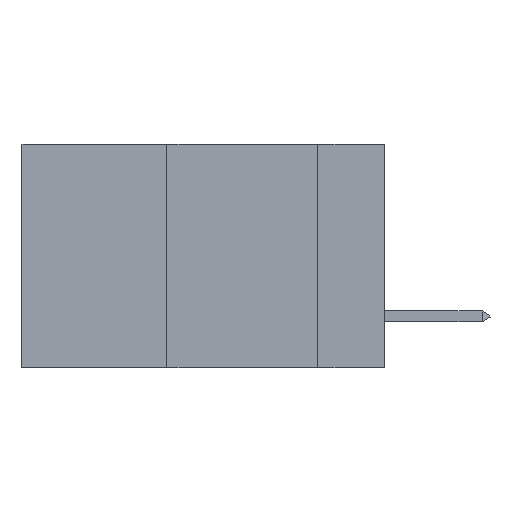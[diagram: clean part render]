
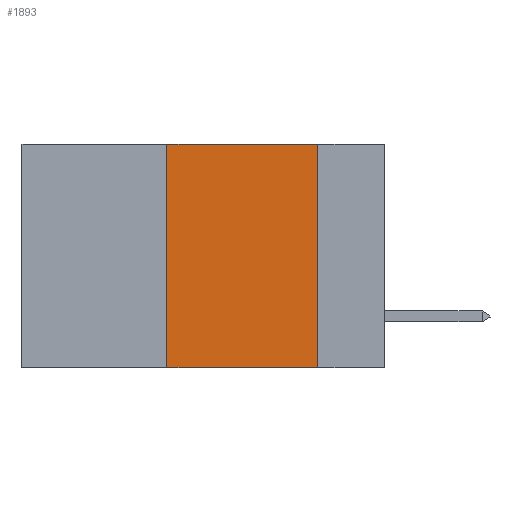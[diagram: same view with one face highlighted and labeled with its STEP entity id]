
A CAD part, left-side view. The second image highlights one B-rep face of the part: STEP entity #1893.
In plain terms, the highlighted planar face has unit normal (-1, 0, 0).
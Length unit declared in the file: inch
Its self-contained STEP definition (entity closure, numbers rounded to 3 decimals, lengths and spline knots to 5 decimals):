
#67 = ORIENTED_EDGE ( 'NONE', *, *, #1870, .F. ) ;
#331 = CARTESIAN_POINT ( 'NONE',  ( 0., 0.36, 0. ) ) ;
#448 = ORIENTED_EDGE ( 'NONE', *, *, #15491, .T. ) ;
#870 = VECTOR ( 'NONE', #1427, 39.37008 ) ;
#1427 = DIRECTION ( 'NONE',  ( 0., -1., 0. ) ) ;
#1555 = DIRECTION ( 'NONE',  ( 0., 0., 1. ) ) ;
#1618 = FACE_OUTER_BOUND ( 'NONE', #8581, .T. ) ;
#1870 = EDGE_CURVE ( 'NONE', #8998, #3329, #5524, .T. ) ;
#1893 = ADVANCED_FACE ( 'NONE', ( #1618 ), #5859, .F. ) ;
#2208 = VECTOR ( 'NONE', #4569, 39.37008 ) ;
#2362 = DIRECTION ( 'NONE',  ( 0., 0., -1. ) ) ;
#3329 = VERTEX_POINT ( 'NONE', #5149 ) ;
#3379 = VERTEX_POINT ( 'NONE', #7198 ) ;
#4250 = EDGE_CURVE ( 'NONE', #6754, #3379, #15057, .T. ) ;
#4335 = LINE ( 'NONE', #10246, #870 ) ;
#4569 = DIRECTION ( 'NONE',  ( 0., -1., 0. ) ) ;
#5149 = CARTESIAN_POINT ( 'NONE',  ( 0., 0.11, -0.37 ) ) ;
#5524 = LINE ( 'NONE', #6118, #9192 ) ;
#5765 = CARTESIAN_POINT ( 'NONE',  ( 0., 0.6, 0. ) ) ;
#5859 = PLANE ( 'NONE',  #11599 ) ;
#5936 = DIRECTION ( 'NONE',  ( 1., 0., 0. ) ) ;
#6118 = CARTESIAN_POINT ( 'NONE',  ( 0., 0.11, 0. ) ) ;
#6259 = DIRECTION ( 'NONE',  ( 0., 0., -1. ) ) ;
#6754 = VERTEX_POINT ( 'NONE', #14789 ) ;
#7198 = CARTESIAN_POINT ( 'NONE',  ( 0., 0.36, 0. ) ) ;
#7748 = EDGE_CURVE ( 'NONE', #3379, #8998, #9362, .T. ) ;
#8167 = ORIENTED_EDGE ( 'NONE', *, *, #4250, .F. ) ;
#8577 = VECTOR ( 'NONE', #1555, 39.37008 ) ;
#8581 = EDGE_LOOP ( 'NONE', ( #67, #15544, #8167, #448 ) ) ;
#8998 = VERTEX_POINT ( 'NONE', #9436 ) ;
#9192 = VECTOR ( 'NONE', #6259, 39.37008 ) ;
#9362 = LINE ( 'NONE', #11936, #2208 ) ;
#9436 = CARTESIAN_POINT ( 'NONE',  ( 0., 0.11, 0. ) ) ;
#10246 = CARTESIAN_POINT ( 'NONE',  ( 0., 0.6, -0.37 ) ) ;
#11599 = AXIS2_PLACEMENT_3D ( 'NONE', #5765, #5936, #2362 ) ;
#11936 = CARTESIAN_POINT ( 'NONE',  ( 0., 0.6, 0. ) ) ;
#14789 = CARTESIAN_POINT ( 'NONE',  ( 0., 0.36, -0.37 ) ) ;
#15057 = LINE ( 'NONE', #331, #8577 ) ;
#15491 = EDGE_CURVE ( 'NONE', #6754, #3329, #4335, .T. ) ;
#15544 = ORIENTED_EDGE ( 'NONE', *, *, #7748, .F. ) ;
